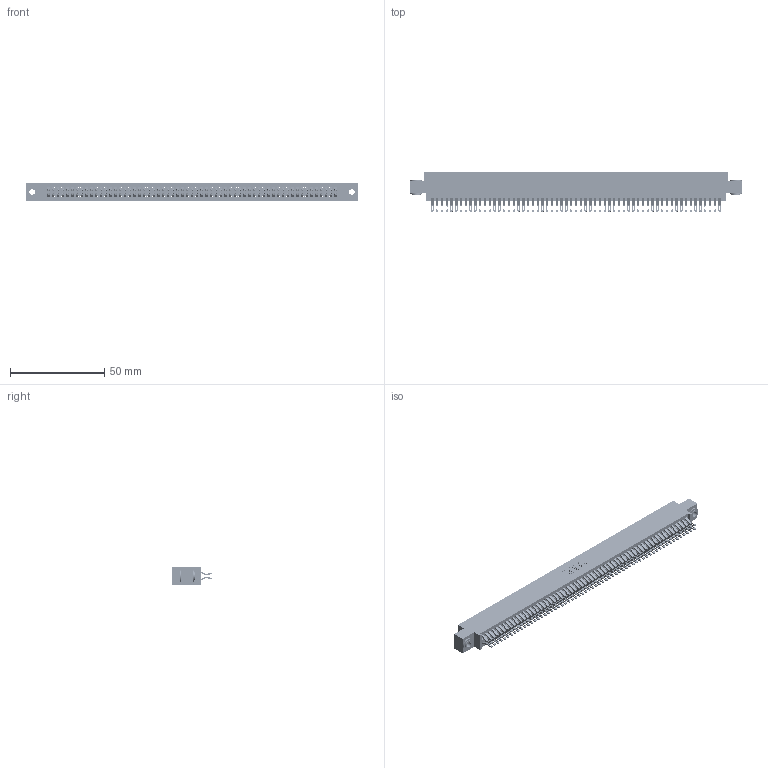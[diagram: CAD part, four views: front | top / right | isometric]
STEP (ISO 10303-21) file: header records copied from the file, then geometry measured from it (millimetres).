
FILE_DESCRIPTION (( 'STEP AP203' ), '1' );
FILE_NAME ('395-122-555-803.STEP', '2019-10-28T08:53:44', ( '' ), ( '' ), 'SwSTEP 2.0', 'SolidWorks 2016', '' );
FILE_SCHEMA (( 'CONFIG_CONTROL_DESIGN' ));
Length unit declared in the file: inch
Products named in the file (4): 345 Part_0.170 Offset - 0.156 Dia-TH; 345-292-001_555 Tail; 345-250-002_345-250-002-102; 395-122-555-803
Assembly tree (125 placements, depth 2):
  395-122-555-803
    345 Part_0.170 Offset - 0.156 Dia-TH
    345-292-001_555 Tail  x122
    345-250-002_345-250-002-102  x2
Bounding box: 176.15 x 21.13 x 9.4 mm (x, y, z)
Volume: 17547.5 mm3; surface area: 27885.3 mm2
Topology: 125 solids, 125 shells, 7000 faces, 22023 edges, 14678 vertices
Faces by surface type: plane 3876, cylinder 3116, cone 8
Entity records: 46412 total; most frequent: CARTESIAN_POINT 7773, ORIENTED_EDGE 7670, DIRECTION 6829, EDGE_CURVE 3835, VECTOR 3415, LINE 3415, VERTEX_POINT 2554, AXIS2_PLACEMENT_3D 1707
